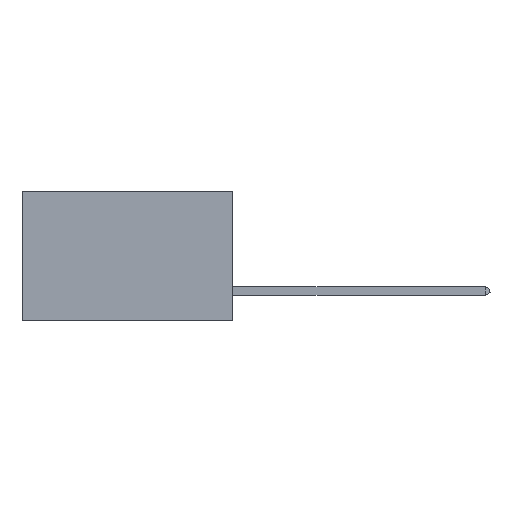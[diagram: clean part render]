
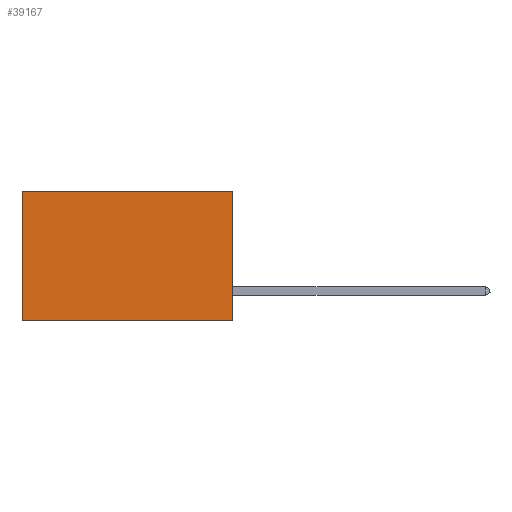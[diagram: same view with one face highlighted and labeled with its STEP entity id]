
A CAD part, left-side view. The second image highlights one B-rep face of the part: STEP entity #39167.
In plain terms, the highlighted planar face has unit normal (-1, 0, 0).
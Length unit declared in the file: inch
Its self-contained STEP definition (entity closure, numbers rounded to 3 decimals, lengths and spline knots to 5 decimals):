
#388 = ORIENTED_EDGE ( 'NONE', *, *, #18985, .F. ) ;
#2199 = ORIENTED_EDGE ( 'NONE', *, *, #31609, .F. ) ;
#4266 = CARTESIAN_POINT ( 'NONE',  ( 0.2875, 0., 0. ) ) ;
#4805 = VERTEX_POINT ( 'NONE', #4266 ) ;
#7248 = DIRECTION ( 'NONE',  ( 0., 1., 0. ) ) ;
#8909 = DIRECTION ( 'NONE',  ( 0., 0., -1. ) ) ;
#9484 = CARTESIAN_POINT ( 'NONE',  ( 0.2875, 0.6, 0. ) ) ;
#9546 = VECTOR ( 'NONE', #13032, 39.37008 ) ;
#12089 = VERTEX_POINT ( 'NONE', #38591 ) ;
#12347 = CARTESIAN_POINT ( 'NONE',  ( 0.2875, 0., 0. ) ) ;
#12372 = EDGE_CURVE ( 'NONE', #17224, #12089, #41924, .T. ) ;
#13032 = DIRECTION ( 'NONE',  ( 0., 1., 0. ) ) ;
#15639 = EDGE_LOOP ( 'NONE', ( #35830, #388, #2199, #35087 ) ) ;
#17224 = VERTEX_POINT ( 'NONE', #26811 ) ;
#18031 = LINE ( 'NONE', #32408, #41111 ) ;
#18985 = EDGE_CURVE ( 'NONE', #38232, #12089, #19106, .T. ) ;
#18994 = LINE ( 'NONE', #19685, #24759 ) ;
#19106 = LINE ( 'NONE', #34729, #9546 ) ;
#19685 = CARTESIAN_POINT ( 'NONE',  ( 0.2875, 0., 0. ) ) ;
#23267 = EDGE_CURVE ( 'NONE', #4805, #17224, #18031, .T. ) ;
#24759 = VECTOR ( 'NONE', #30429, 39.37008 ) ;
#25002 = VECTOR ( 'NONE', #42048, 39.37008 ) ;
#25693 = DIRECTION ( 'NONE',  ( 1., 0., 0. ) ) ;
#26811 = CARTESIAN_POINT ( 'NONE',  ( 0.2875, 0.6, 0. ) ) ;
#27300 = CARTESIAN_POINT ( 'NONE',  ( 0.2875, 0., -0.37 ) ) ;
#30429 = DIRECTION ( 'NONE',  ( 0., 0., -1. ) ) ;
#31609 = EDGE_CURVE ( 'NONE', #4805, #38232, #18994, .T. ) ;
#32408 = CARTESIAN_POINT ( 'NONE',  ( 0.2875, 0., 0. ) ) ;
#34729 = CARTESIAN_POINT ( 'NONE',  ( 0.2875, 0., -0.37 ) ) ;
#35087 = ORIENTED_EDGE ( 'NONE', *, *, #23267, .T. ) ;
#35124 = FACE_OUTER_BOUND ( 'NONE', #15639, .T. ) ;
#35830 = ORIENTED_EDGE ( 'NONE', *, *, #12372, .T. ) ;
#36720 = PLANE ( 'NONE',  #44173 ) ;
#38232 = VERTEX_POINT ( 'NONE', #27300 ) ;
#38591 = CARTESIAN_POINT ( 'NONE',  ( 0.2875, 0.6, -0.37 ) ) ;
#39167 = ADVANCED_FACE ( 'NONE', ( #35124 ), #36720, .F. ) ;
#41111 = VECTOR ( 'NONE', #7248, 39.37008 ) ;
#41924 = LINE ( 'NONE', #9484, #25002 ) ;
#42048 = DIRECTION ( 'NONE',  ( 0., 0., -1. ) ) ;
#44173 = AXIS2_PLACEMENT_3D ( 'NONE', #12347, #25693, #8909 ) ;
